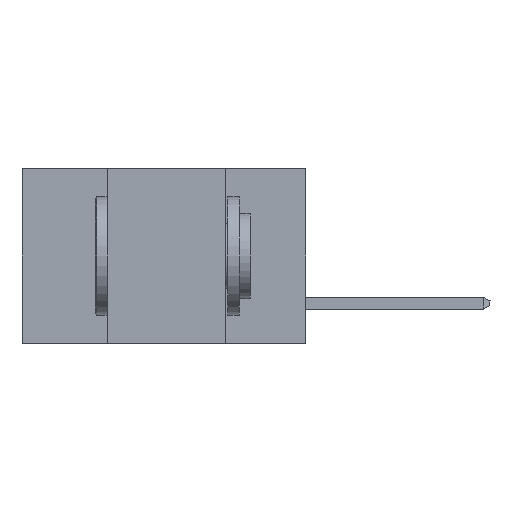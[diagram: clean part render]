
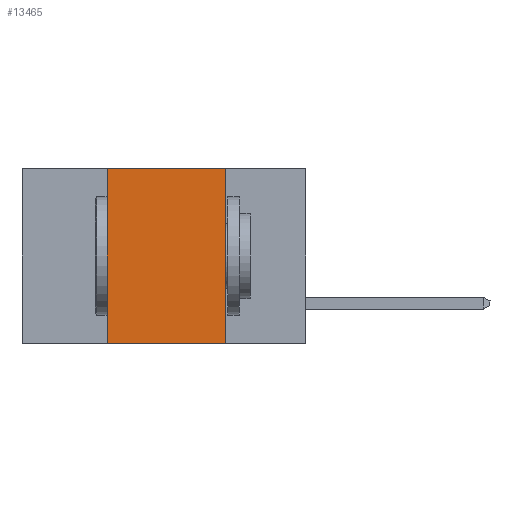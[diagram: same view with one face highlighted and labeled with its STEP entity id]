
A CAD part, left-side view. The second image highlights one B-rep face of the part: STEP entity #13465.
In plain terms, the highlighted planar face has unit normal (-1, 0, 0).
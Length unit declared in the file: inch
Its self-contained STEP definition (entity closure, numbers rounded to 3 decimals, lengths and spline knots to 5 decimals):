
#523 = CARTESIAN_POINT ( 'NONE',  ( 0., 0.17, -0.37 ) ) ;
#1021 = CARTESIAN_POINT ( 'NONE',  ( 0., 0.6, -0.37 ) ) ;
#1711 = ORIENTED_EDGE ( 'NONE', *, *, #5743, .F. ) ;
#2393 = CARTESIAN_POINT ( 'NONE',  ( 0., 0.42, -0.37 ) ) ;
#3979 = EDGE_LOOP ( 'NONE', ( #1711, #10734, #21617, #15743 ) ) ;
#4478 = VECTOR ( 'NONE', #10762, 39.37008 ) ;
#4708 = CARTESIAN_POINT ( 'NONE',  ( 0., 0.17, 0. ) ) ;
#5363 = FACE_OUTER_BOUND ( 'NONE', #3979, .T. ) ;
#5498 = EDGE_CURVE ( 'NONE', #13369, #20373, #9782, .T. ) ;
#5743 = EDGE_CURVE ( 'NONE', #11657, #10864, #17212, .T. ) ;
#5873 = VECTOR ( 'NONE', #6471, 39.37008 ) ;
#6471 = DIRECTION ( 'NONE',  ( 0., 0., 1. ) ) ;
#7172 = AXIS2_PLACEMENT_3D ( 'NONE', #12520, #12084, #9023 ) ;
#7370 = PLANE ( 'NONE',  #7172 ) ;
#9023 = DIRECTION ( 'NONE',  ( 0., 0., -1. ) ) ;
#9189 = DIRECTION ( 'NONE',  ( 0., -1., 0. ) ) ;
#9782 = LINE ( 'NONE', #16341, #5873 ) ;
#9929 = LINE ( 'NONE', #1021, #12760 ) ;
#10734 = ORIENTED_EDGE ( 'NONE', *, *, #15802, .F. ) ;
#10762 = DIRECTION ( 'NONE',  ( 0., 0., -1. ) ) ;
#10864 = VERTEX_POINT ( 'NONE', #21568 ) ;
#11657 = VERTEX_POINT ( 'NONE', #4708 ) ;
#12084 = DIRECTION ( 'NONE',  ( 1., 0., 0. ) ) ;
#12520 = CARTESIAN_POINT ( 'NONE',  ( 0., 0.6, 0. ) ) ;
#12760 = VECTOR ( 'NONE', #12795, 39.37008 ) ;
#12795 = DIRECTION ( 'NONE',  ( 0., -1., 0. ) ) ;
#13369 = VERTEX_POINT ( 'NONE', #2393 ) ;
#13465 = ADVANCED_FACE ( 'NONE', ( #5363 ), #7370, .F. ) ;
#15743 = ORIENTED_EDGE ( 'NONE', *, *, #17798, .T. ) ;
#15744 = LINE ( 'NONE', #17597, #17910 ) ;
#15802 = EDGE_CURVE ( 'NONE', #20373, #11657, #15744, .T. ) ;
#16341 = CARTESIAN_POINT ( 'NONE',  ( 0., 0.42, -0.37 ) ) ;
#17212 = LINE ( 'NONE', #523, #4478 ) ;
#17597 = CARTESIAN_POINT ( 'NONE',  ( 0., 0.6, 0. ) ) ;
#17798 = EDGE_CURVE ( 'NONE', #13369, #10864, #9929, .T. ) ;
#17910 = VECTOR ( 'NONE', #9189, 39.37008 ) ;
#20373 = VERTEX_POINT ( 'NONE', #21233 ) ;
#21233 = CARTESIAN_POINT ( 'NONE',  ( 0., 0.42, 0. ) ) ;
#21568 = CARTESIAN_POINT ( 'NONE',  ( 0., 0.17, -0.37 ) ) ;
#21617 = ORIENTED_EDGE ( 'NONE', *, *, #5498, .F. ) ;
